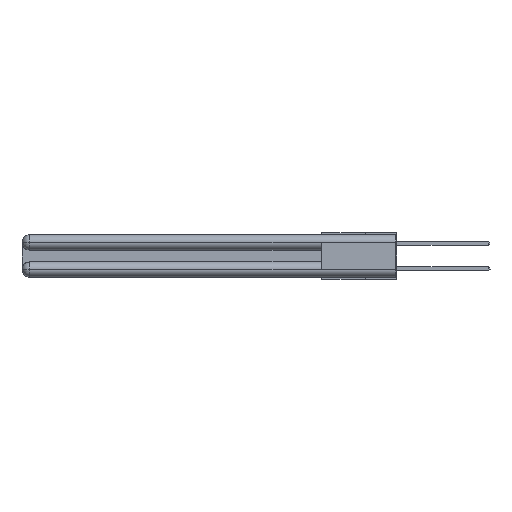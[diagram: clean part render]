
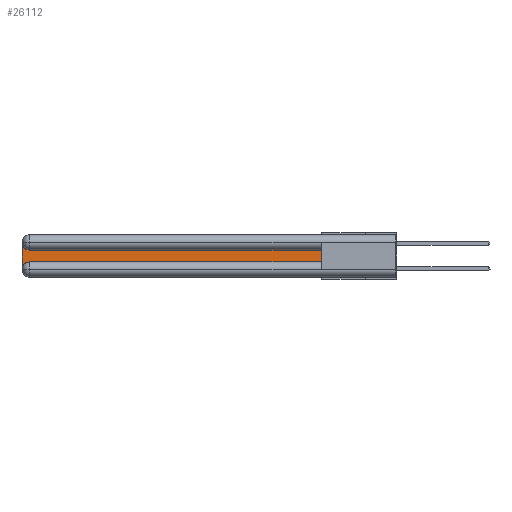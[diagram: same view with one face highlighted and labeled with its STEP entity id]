
A CAD part, left-side view. The second image highlights one B-rep face of the part: STEP entity #26112.
In plain terms, the highlighted planar face has unit normal (-1, 0, 0).
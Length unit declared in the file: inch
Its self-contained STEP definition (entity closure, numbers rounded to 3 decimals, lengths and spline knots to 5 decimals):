
#1424 = EDGE_CURVE ( 'NONE', #29803, #25556, #16835, .T. ) ;
#1511 = CIRCLE ( 'NONE', #14503, 0.06 ) ;
#1939 = CARTESIAN_POINT ( 'NONE',  ( 0.075, 3., -0.0625 ) ) ;
#3096 = CARTESIAN_POINT ( 'NONE',  ( 0.075, 3., -0.2775 ) ) ;
#3299 = DIRECTION ( 'NONE',  ( 1., 0., 0. ) ) ;
#3886 = CARTESIAN_POINT ( 'NONE',  ( 0.075, 0.6, -0.2175 ) ) ;
#5034 = LINE ( 'NONE', #26713, #6902 ) ;
#6056 = EDGE_CURVE ( 'NONE', #14296, #14111, #1511, .T. ) ;
#6473 = ORIENTED_EDGE ( 'NONE', *, *, #29508, .T. ) ;
#6816 = EDGE_CURVE ( 'NONE', #10037, #14296, #28935, .T. ) ;
#6902 = VECTOR ( 'NONE', #27437, 39.37008 ) ;
#7743 = CARTESIAN_POINT ( 'NONE',  ( 0.075, 2.94, -0.2175 ) ) ;
#7832 = CARTESIAN_POINT ( 'NONE',  ( 0.075, 0.6, -0.2175 ) ) ;
#7849 = VERTEX_POINT ( 'NONE', #18422 ) ;
#8828 = ORIENTED_EDGE ( 'NONE', *, *, #11802, .T. ) ;
#10037 = VERTEX_POINT ( 'NONE', #1939 ) ;
#10195 = DIRECTION ( 'NONE',  ( 1., 0., 0. ) ) ;
#11802 = EDGE_CURVE ( 'NONE', #14111, #29803, #30784, .T. ) ;
#13118 = EDGE_CURVE ( 'NONE', #25556, #7849, #5034, .T. ) ;
#14111 = VERTEX_POINT ( 'NONE', #7743 ) ;
#14296 = VERTEX_POINT ( 'NONE', #3096 ) ;
#14503 = AXIS2_PLACEMENT_3D ( 'NONE', #29734, #10195, #15056 ) ;
#14728 = CARTESIAN_POINT ( 'NONE',  ( 0.075, 3., -0.2175 ) ) ;
#15056 = DIRECTION ( 'NONE',  ( 0., 0., -1. ) ) ;
#16820 = DIRECTION ( 'NONE',  ( 0., 0., 1. ) ) ;
#16835 = LINE ( 'NONE', #17054, #25679 ) ;
#17054 = CARTESIAN_POINT ( 'NONE',  ( 0.075, 0.6, -0.2175 ) ) ;
#18106 = DIRECTION ( 'NONE',  ( 1., 0., 0. ) ) ;
#18144 = ORIENTED_EDGE ( 'NONE', *, *, #13118, .T. ) ;
#18422 = CARTESIAN_POINT ( 'NONE',  ( 0.075, 2.94, -0.1225 ) ) ;
#21281 = ORIENTED_EDGE ( 'NONE', *, *, #6816, .T. ) ;
#21583 = FACE_OUTER_BOUND ( 'NONE', #31218, .T. ) ;
#22744 = PLANE ( 'NONE',  #25030 ) ;
#23305 = CARTESIAN_POINT ( 'NONE',  ( 0.075, 0.6, -0.1225 ) ) ;
#23459 = AXIS2_PLACEMENT_3D ( 'NONE', #28008, #18106, #25505 ) ;
#24126 = CIRCLE ( 'NONE', #23459, 0.06 ) ;
#25030 = AXIS2_PLACEMENT_3D ( 'NONE', #27808, #3299, #30400 ) ;
#25489 = VECTOR ( 'NONE', #29847, 39.37008 ) ;
#25505 = DIRECTION ( 'NONE',  ( 0., 0., -1. ) ) ;
#25556 = VERTEX_POINT ( 'NONE', #23305 ) ;
#25611 = ORIENTED_EDGE ( 'NONE', *, *, #1424, .T. ) ;
#25679 = VECTOR ( 'NONE', #16820, 39.37008 ) ;
#26112 = ADVANCED_FACE ( 'NONE', ( #21583 ), #22744, .F. ) ;
#26659 = VECTOR ( 'NONE', #29507, 39.37008 ) ;
#26713 = CARTESIAN_POINT ( 'NONE',  ( 0.075, 0.6, -0.1225 ) ) ;
#27437 = DIRECTION ( 'NONE',  ( 0., 1., 0. ) ) ;
#27808 = CARTESIAN_POINT ( 'NONE',  ( 0.075, 3., -0.1225 ) ) ;
#28008 = CARTESIAN_POINT ( 'NONE',  ( 0.075, 2.94, -0.0625 ) ) ;
#28935 = LINE ( 'NONE', #14728, #26659 ) ;
#29356 = ORIENTED_EDGE ( 'NONE', *, *, #6056, .T. ) ;
#29507 = DIRECTION ( 'NONE',  ( 0., 0., -1. ) ) ;
#29508 = EDGE_CURVE ( 'NONE', #7849, #10037, #24126, .T. ) ;
#29734 = CARTESIAN_POINT ( 'NONE',  ( 0.075, 2.94, -0.2775 ) ) ;
#29803 = VERTEX_POINT ( 'NONE', #3886 ) ;
#29847 = DIRECTION ( 'NONE',  ( 0., -1., 0. ) ) ;
#30400 = DIRECTION ( 'NONE',  ( 0., 0., -1. ) ) ;
#30784 = LINE ( 'NONE', #7832, #25489 ) ;
#31218 = EDGE_LOOP ( 'NONE', ( #18144, #6473, #21281, #29356, #8828, #25611 ) ) ;
